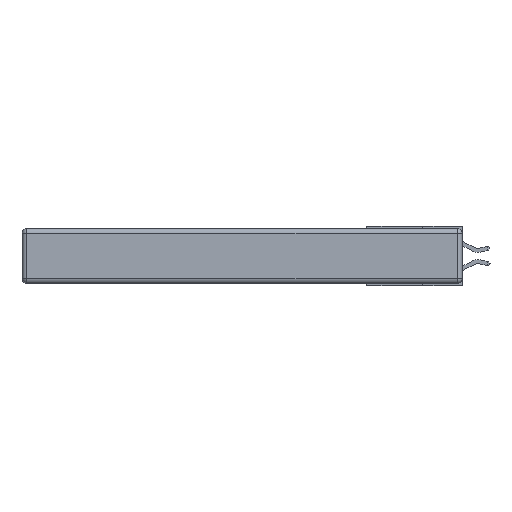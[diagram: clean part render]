
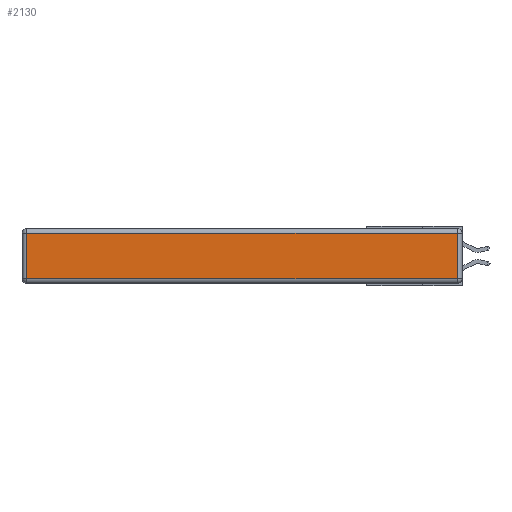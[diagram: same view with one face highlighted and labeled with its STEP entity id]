
A CAD part, left-side view. The second image highlights one B-rep face of the part: STEP entity #2130.
In plain terms, the highlighted planar face has unit normal (-1, 0, 0).
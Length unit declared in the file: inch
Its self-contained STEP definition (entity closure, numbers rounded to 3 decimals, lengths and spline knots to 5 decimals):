
#3 = CARTESIAN_POINT ( 'NONE',  ( 0., 0.03, -0.03 ) ) ;
#173 = CARTESIAN_POINT ( 'NONE',  ( 0., 2.72, -0.343 ) ) ;
#432 = CARTESIAN_POINT ( 'NONE',  ( 0., 2.72, -0.313 ) ) ;
#1745 = EDGE_CURVE ( 'NONE', #9348, #3936, #8581, .T. ) ;
#2130 = ADVANCED_FACE ( 'NONE', ( #10633 ), #3173, .T. ) ;
#2191 = VERTEX_POINT ( 'NONE', #432 ) ;
#2282 = EDGE_CURVE ( 'NONE', #6605, #9348, #5454, .T. ) ;
#2777 = EDGE_CURVE ( 'NONE', #3936, #2191, #9680, .T. ) ;
#3173 = PLANE ( 'NONE',  #11761 ) ;
#3494 = LINE ( 'NONE', #8973, #8496 ) ;
#3544 = DIRECTION ( 'NONE',  ( 0., 1., 0. ) ) ;
#3936 = VERTEX_POINT ( 'NONE', #5724 ) ;
#4243 = DIRECTION ( 'NONE',  ( 0., 0., -1. ) ) ;
#5454 = LINE ( 'NONE', #7679, #12783 ) ;
#5467 = ORIENTED_EDGE ( 'NONE', *, *, #2282, .T. ) ;
#5724 = CARTESIAN_POINT ( 'NONE',  ( 0., 2.72, -0.03 ) ) ;
#6605 = VERTEX_POINT ( 'NONE', #8815 ) ;
#6710 = DIRECTION ( 'NONE',  ( 0., 0., 1. ) ) ;
#7152 = CARTESIAN_POINT ( 'NONE',  ( 0., 0., -0.343 ) ) ;
#7628 = VECTOR ( 'NONE', #4243, 39.37008 ) ;
#7679 = CARTESIAN_POINT ( 'NONE',  ( 0., 0.03, -0.343 ) ) ;
#8496 = VECTOR ( 'NONE', #12852, 39.37008 ) ;
#8581 = LINE ( 'NONE', #12532, #11400 ) ;
#8815 = CARTESIAN_POINT ( 'NONE',  ( 0., 0.03, -0.313 ) ) ;
#8973 = CARTESIAN_POINT ( 'NONE',  ( 0., 0., -0.313 ) ) ;
#9252 = ORIENTED_EDGE ( 'NONE', *, *, #2777, .T. ) ;
#9308 = ORIENTED_EDGE ( 'NONE', *, *, #1745, .T. ) ;
#9348 = VERTEX_POINT ( 'NONE', #3 ) ;
#9680 = LINE ( 'NONE', #173, #7628 ) ;
#9723 = EDGE_CURVE ( 'NONE', #2191, #6605, #3494, .T. ) ;
#9904 = ORIENTED_EDGE ( 'NONE', *, *, #9723, .T. ) ;
#10280 = DIRECTION ( 'NONE',  ( -1., 0., 0. ) ) ;
#10633 = FACE_OUTER_BOUND ( 'NONE', #10661, .T. ) ;
#10661 = EDGE_LOOP ( 'NONE', ( #9904, #5467, #9308, #9252 ) ) ;
#11400 = VECTOR ( 'NONE', #3544, 39.37008 ) ;
#11761 = AXIS2_PLACEMENT_3D ( 'NONE', #7152, #10280, #12259 ) ;
#12259 = DIRECTION ( 'NONE',  ( 0., 0., 1. ) ) ;
#12532 = CARTESIAN_POINT ( 'NONE',  ( 0., 2.75, -0.03 ) ) ;
#12783 = VECTOR ( 'NONE', #6710, 39.37008 ) ;
#12852 = DIRECTION ( 'NONE',  ( 0., -1., 0. ) ) ;
